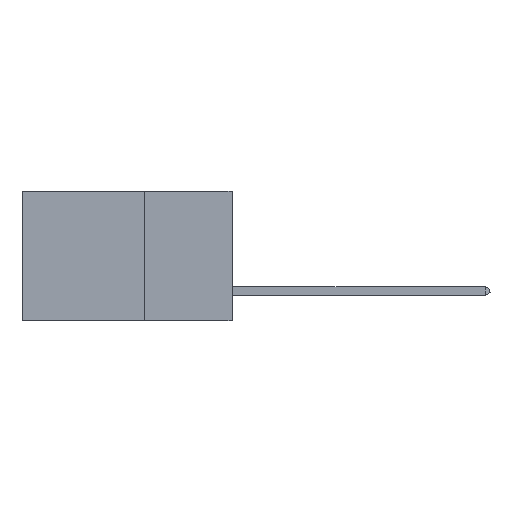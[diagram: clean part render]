
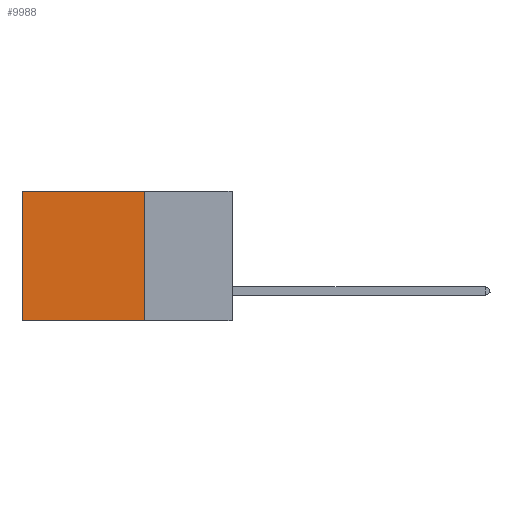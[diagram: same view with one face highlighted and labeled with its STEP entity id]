
A CAD part, left-side view. The second image highlights one B-rep face of the part: STEP entity #9988.
In plain terms, the highlighted planar face has unit normal (-1, 0, 0).
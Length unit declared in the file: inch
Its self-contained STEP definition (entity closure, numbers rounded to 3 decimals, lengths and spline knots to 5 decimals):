
#213 = DIRECTION ( 'NONE',  ( 1., 0., 0. ) ) ;
#642 = ORIENTED_EDGE ( 'NONE', *, *, #15941, .T. ) ;
#1519 = CARTESIAN_POINT ( 'NONE',  ( 0.2875, 0.25, 0. ) ) ;
#1530 = CARTESIAN_POINT ( 'NONE',  ( 0.2875, 0.6, 0. ) ) ;
#1925 = PLANE ( 'NONE',  #16714 ) ;
#2999 = EDGE_CURVE ( 'NONE', #4358, #15051, #17163, .T. ) ;
#3116 = LINE ( 'NONE', #17171, #3618 ) ;
#3271 = DIRECTION ( 'NONE',  ( 0., 1., 0. ) ) ;
#3618 = VECTOR ( 'NONE', #10109, 39.37008 ) ;
#4338 = ORIENTED_EDGE ( 'NONE', *, *, #2999, .F. ) ;
#4358 = VERTEX_POINT ( 'NONE', #13329 ) ;
#7197 = DIRECTION ( 'NONE',  ( 0., 0., -1. ) ) ;
#7807 = LINE ( 'NONE', #14764, #17187 ) ;
#8036 = CARTESIAN_POINT ( 'NONE',  ( 0.2875, 0.6, -0.37 ) ) ;
#8049 = VERTEX_POINT ( 'NONE', #8036 ) ;
#8486 = DIRECTION ( 'NONE',  ( 0., 0., -1. ) ) ;
#9988 = ADVANCED_FACE ( 'NONE', ( #20989 ), #1925, .F. ) ;
#10109 = DIRECTION ( 'NONE',  ( 0., 1., 0. ) ) ;
#10338 = EDGE_LOOP ( 'NONE', ( #642, #15285, #4338, #16599 ) ) ;
#11104 = VECTOR ( 'NONE', #3271, 39.37008 ) ;
#11455 = EDGE_CURVE ( 'NONE', #4358, #19139, #3116, .T. ) ;
#11623 = CARTESIAN_POINT ( 'NONE',  ( 0.2875, 0.25, -0.37 ) ) ;
#13329 = CARTESIAN_POINT ( 'NONE',  ( 0.2875, 0.25, 0. ) ) ;
#13450 = LINE ( 'NONE', #11623, #11104 ) ;
#14764 = CARTESIAN_POINT ( 'NONE',  ( 0.2875, 0.6, 0. ) ) ;
#15051 = VERTEX_POINT ( 'NONE', #20177 ) ;
#15285 = ORIENTED_EDGE ( 'NONE', *, *, #18745, .F. ) ;
#15405 = VECTOR ( 'NONE', #8486, 39.37008 ) ;
#15853 = CARTESIAN_POINT ( 'NONE',  ( 0.2875, 0.25, 0. ) ) ;
#15941 = EDGE_CURVE ( 'NONE', #19139, #8049, #7807, .T. ) ;
#16599 = ORIENTED_EDGE ( 'NONE', *, *, #11455, .T. ) ;
#16714 = AXIS2_PLACEMENT_3D ( 'NONE', #15853, #213, #7197 ) ;
#17163 = LINE ( 'NONE', #1519, #15405 ) ;
#17171 = CARTESIAN_POINT ( 'NONE',  ( 0.2875, 0.25, 0. ) ) ;
#17187 = VECTOR ( 'NONE', #21735, 39.37008 ) ;
#18745 = EDGE_CURVE ( 'NONE', #15051, #8049, #13450, .T. ) ;
#19139 = VERTEX_POINT ( 'NONE', #1530 ) ;
#20177 = CARTESIAN_POINT ( 'NONE',  ( 0.2875, 0.25, -0.37 ) ) ;
#20989 = FACE_OUTER_BOUND ( 'NONE', #10338, .T. ) ;
#21735 = DIRECTION ( 'NONE',  ( 0., 0., -1. ) ) ;
